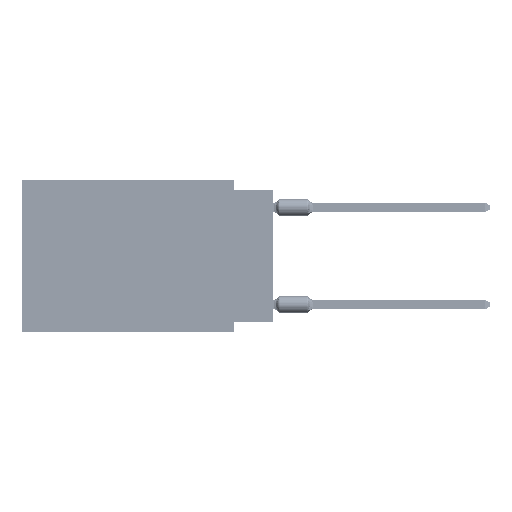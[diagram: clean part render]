
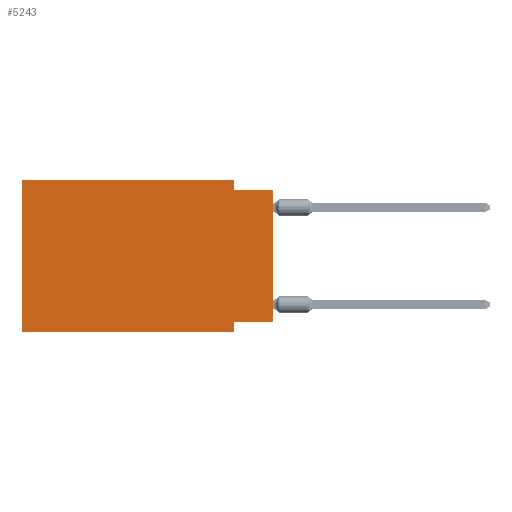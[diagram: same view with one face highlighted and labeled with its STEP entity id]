
A CAD part, left-side view. The second image highlights one B-rep face of the part: STEP entity #5243.
In plain terms, the highlighted planar face has unit normal (-1, 0, 0).
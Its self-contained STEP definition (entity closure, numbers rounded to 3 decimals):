
#2523 = CARTESIAN_POINT ( 'NONE',  ( 0., 0., -9.271 ) ) ;
#4577 = VECTOR ( 'NONE', #7076, 1000. ) ;
#5243 = ADVANCED_FACE ( 'NONE', ( #43842 ), #38286, .F. ) ;
#5355 = CARTESIAN_POINT ( 'NONE',  ( 0., 2.54, -9.271 ) ) ;
#7076 = DIRECTION ( 'NONE',  ( 0., 1., 0. ) ) ;
#7889 = VERTEX_POINT ( 'NONE', #60569 ) ;
#8655 = DIRECTION ( 'NONE',  ( 0., 0., 1. ) ) ;
#9123 = CARTESIAN_POINT ( 'NONE',  ( 0., 16.383, 0. ) ) ;
#12509 = EDGE_CURVE ( 'NONE', #23418, #51990, #18576, .T. ) ;
#13640 = CARTESIAN_POINT ( 'NONE',  ( 0., 16.383, 0. ) ) ;
#13771 = CARTESIAN_POINT ( 'NONE',  ( 0., 2.54, 0. ) ) ;
#14642 = AXIS2_PLACEMENT_3D ( 'NONE', #60898, #38656, #65714 ) ;
#14907 = CARTESIAN_POINT ( 'NONE',  ( 0., 16.383, 0. ) ) ;
#15111 = CARTESIAN_POINT ( 'NONE',  ( 0., 0., -0.635 ) ) ;
#15416 = VECTOR ( 'NONE', #26004, 1000. ) ;
#16303 = CARTESIAN_POINT ( 'NONE',  ( 0., 2.54, 0. ) ) ;
#18576 = LINE ( 'NONE', #62676, #4577 ) ;
#19878 = EDGE_CURVE ( 'NONE', #23418, #22961, #54953, .T. ) ;
#20473 = DIRECTION ( 'NONE',  ( 0., -1., 0. ) ) ;
#21796 = LINE ( 'NONE', #44016, #69188 ) ;
#22961 = VERTEX_POINT ( 'NONE', #15111 ) ;
#22969 = ORIENTED_EDGE ( 'NONE', *, *, #12509, .F. ) ;
#23418 = VERTEX_POINT ( 'NONE', #2523 ) ;
#24798 = ORIENTED_EDGE ( 'NONE', *, *, #48712, .F. ) ;
#26004 = DIRECTION ( 'NONE',  ( 0., -1., 0. ) ) ;
#26805 = EDGE_LOOP ( 'NONE', ( #42025, #46243, #63469, #58522, #24798, #40756, #66719, #22969 ) ) ;
#28124 = LINE ( 'NONE', #16303, #33620 ) ;
#30528 = VECTOR ( 'NONE', #49112, 1000. ) ;
#30883 = VECTOR ( 'NONE', #20473, 1000. ) ;
#31831 = VERTEX_POINT ( 'NONE', #44436 ) ;
#32416 = LINE ( 'NONE', #37250, #30528 ) ;
#33310 = DIRECTION ( 'NONE',  ( 0., 0., -1. ) ) ;
#33620 = VECTOR ( 'NONE', #33310, 1000. ) ;
#33967 = VERTEX_POINT ( 'NONE', #13771 ) ;
#36788 = CARTESIAN_POINT ( 'NONE',  ( 0., 0., 0. ) ) ;
#37250 = CARTESIAN_POINT ( 'NONE',  ( 0., 2.54, -9.906 ) ) ;
#38286 = PLANE ( 'NONE',  #14642 ) ;
#38554 = VECTOR ( 'NONE', #54317, 1000. ) ;
#38656 = DIRECTION ( 'NONE',  ( 1., 0., 0. ) ) ;
#38820 = DIRECTION ( 'NONE',  ( 0., -1., 0. ) ) ;
#40756 = ORIENTED_EDGE ( 'NONE', *, *, #71210, .T. ) ;
#42025 = ORIENTED_EDGE ( 'NONE', *, *, #19878, .T. ) ;
#43313 = VERTEX_POINT ( 'NONE', #55738 ) ;
#43842 = FACE_OUTER_BOUND ( 'NONE', #26805, .T. ) ;
#43972 = VERTEX_POINT ( 'NONE', #13640 ) ;
#44016 = CARTESIAN_POINT ( 'NONE',  ( 0., 16.383, -9.906 ) ) ;
#44436 = CARTESIAN_POINT ( 'NONE',  ( 0., 16.383, -9.906 ) ) ;
#45161 = VECTOR ( 'NONE', #8655, 1000. ) ;
#46243 = ORIENTED_EDGE ( 'NONE', *, *, #63938, .F. ) ;
#48620 = LINE ( 'NONE', #71203, #30883 ) ;
#48712 = EDGE_CURVE ( 'NONE', #31831, #43972, #59881, .T. ) ;
#49112 = DIRECTION ( 'NONE',  ( 0., 0., -1. ) ) ;
#51990 = VERTEX_POINT ( 'NONE', #5355 ) ;
#54317 = DIRECTION ( 'NONE',  ( 0., 0., 1. ) ) ;
#54953 = LINE ( 'NONE', #36788, #45161 ) ;
#55644 = LINE ( 'NONE', #14907, #15416 ) ;
#55738 = CARTESIAN_POINT ( 'NONE',  ( 0., 2.54, -0.635 ) ) ;
#58010 = EDGE_CURVE ( 'NONE', #51990, #7889, #32416, .T. ) ;
#58522 = ORIENTED_EDGE ( 'NONE', *, *, #62628, .F. ) ;
#59881 = LINE ( 'NONE', #9123, #38554 ) ;
#60569 = CARTESIAN_POINT ( 'NONE',  ( 0., 2.54, -9.906 ) ) ;
#60898 = CARTESIAN_POINT ( 'NONE',  ( 0., 16.383, 0. ) ) ;
#62628 = EDGE_CURVE ( 'NONE', #43972, #33967, #55644, .T. ) ;
#62676 = CARTESIAN_POINT ( 'NONE',  ( 0., 0., -9.271 ) ) ;
#63469 = ORIENTED_EDGE ( 'NONE', *, *, #69280, .F. ) ;
#63938 = EDGE_CURVE ( 'NONE', #43313, #22961, #48620, .T. ) ;
#65714 = DIRECTION ( 'NONE',  ( 0., 0., -1. ) ) ;
#66719 = ORIENTED_EDGE ( 'NONE', *, *, #58010, .F. ) ;
#69188 = VECTOR ( 'NONE', #38820, 1000. ) ;
#69280 = EDGE_CURVE ( 'NONE', #33967, #43313, #28124, .T. ) ;
#71203 = CARTESIAN_POINT ( 'NONE',  ( 0., 0., -0.635 ) ) ;
#71210 = EDGE_CURVE ( 'NONE', #31831, #7889, #21796, .T. ) ;
